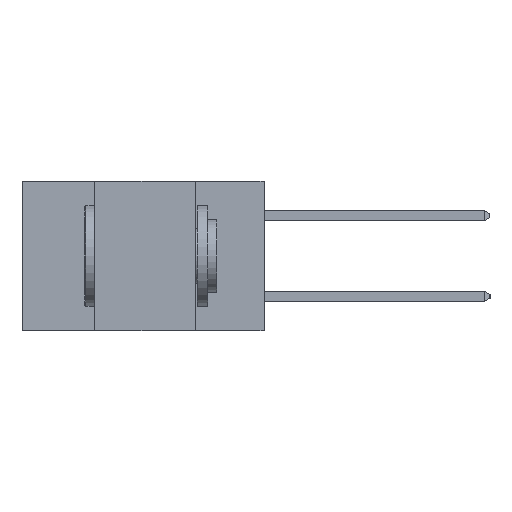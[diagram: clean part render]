
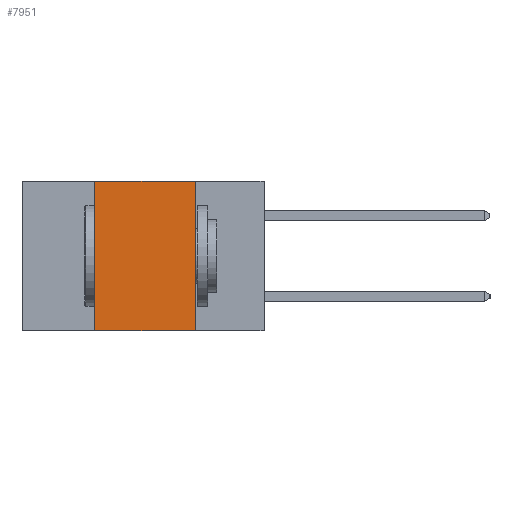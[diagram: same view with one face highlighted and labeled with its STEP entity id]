
A CAD part, left-side view. The second image highlights one B-rep face of the part: STEP entity #7951.
In plain terms, the highlighted planar face has unit normal (-1, 0, 0).
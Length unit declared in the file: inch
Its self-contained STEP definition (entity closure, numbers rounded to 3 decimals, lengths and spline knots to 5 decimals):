
#245 = LINE ( 'NONE', #1488, #9582 ) ;
#470 = VECTOR ( 'NONE', #1966, 39.37008 ) ;
#597 = LINE ( 'NONE', #3404, #8480 ) ;
#1000 = EDGE_LOOP ( 'NONE', ( #7268, #5166, #9710, #5452 ) ) ;
#1098 = EDGE_CURVE ( 'NONE', #8561, #3656, #5059, .T. ) ;
#1234 = EDGE_CURVE ( 'NONE', #6624, #8561, #8102, .T. ) ;
#1488 = CARTESIAN_POINT ( 'NONE',  ( 0., 0.6, -0.37 ) ) ;
#1725 = CARTESIAN_POINT ( 'NONE',  ( 0., 0.6, 0. ) ) ;
#1966 = DIRECTION ( 'NONE',  ( 0., 0., 1. ) ) ;
#2409 = EDGE_CURVE ( 'NONE', #3656, #4778, #597, .T. ) ;
#2449 = DIRECTION ( 'NONE',  ( 0., -1., 0. ) ) ;
#2605 = VECTOR ( 'NONE', #5015, 39.37008 ) ;
#3404 = CARTESIAN_POINT ( 'NONE',  ( 0., 0.17, -0.37 ) ) ;
#3656 = VERTEX_POINT ( 'NONE', #4324 ) ;
#4324 = CARTESIAN_POINT ( 'NONE',  ( 0., 0.17, 0. ) ) ;
#4500 = AXIS2_PLACEMENT_3D ( 'NONE', #10109, #5043, #10879 ) ;
#4778 = VERTEX_POINT ( 'NONE', #8398 ) ;
#5015 = DIRECTION ( 'NONE',  ( 0., -1., 0. ) ) ;
#5043 = DIRECTION ( 'NONE',  ( 1., 0., 0. ) ) ;
#5059 = LINE ( 'NONE', #1725, #2605 ) ;
#5166 = ORIENTED_EDGE ( 'NONE', *, *, #1098, .F. ) ;
#5404 = CARTESIAN_POINT ( 'NONE',  ( 0., 0.42, -0.37 ) ) ;
#5452 = ORIENTED_EDGE ( 'NONE', *, *, #8090, .T. ) ;
#6042 = CARTESIAN_POINT ( 'NONE',  ( 0., 0.42, -0.37 ) ) ;
#6455 = FACE_OUTER_BOUND ( 'NONE', #1000, .T. ) ;
#6624 = VERTEX_POINT ( 'NONE', #5404 ) ;
#7268 = ORIENTED_EDGE ( 'NONE', *, *, #2409, .F. ) ;
#7761 = CARTESIAN_POINT ( 'NONE',  ( 0., 0.42, 0. ) ) ;
#7951 = ADVANCED_FACE ( 'NONE', ( #6455 ), #8544, .F. ) ;
#8090 = EDGE_CURVE ( 'NONE', #6624, #4778, #245, .T. ) ;
#8102 = LINE ( 'NONE', #6042, #470 ) ;
#8398 = CARTESIAN_POINT ( 'NONE',  ( 0., 0.17, -0.37 ) ) ;
#8480 = VECTOR ( 'NONE', #10386, 39.37008 ) ;
#8544 = PLANE ( 'NONE',  #4500 ) ;
#8561 = VERTEX_POINT ( 'NONE', #7761 ) ;
#9582 = VECTOR ( 'NONE', #2449, 39.37008 ) ;
#9710 = ORIENTED_EDGE ( 'NONE', *, *, #1234, .F. ) ;
#10109 = CARTESIAN_POINT ( 'NONE',  ( 0., 0.6, 0. ) ) ;
#10386 = DIRECTION ( 'NONE',  ( 0., 0., -1. ) ) ;
#10879 = DIRECTION ( 'NONE',  ( 0., 0., -1. ) ) ;
